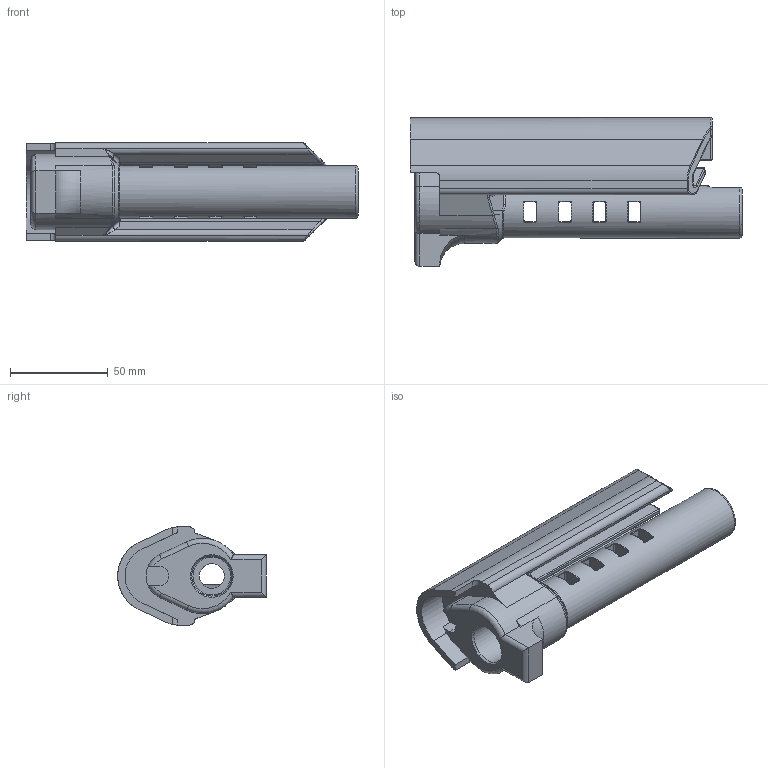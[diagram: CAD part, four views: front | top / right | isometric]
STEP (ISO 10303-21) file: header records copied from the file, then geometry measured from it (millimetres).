
FILE_DESCRIPTION(/* description */ (''),/* implementation_level */ '2;1');
FILE_NAME(/* name */ 'Mount-Cheekrest V2 - Generic.stp',/* time_stamp */ '2021-12-02T15:04:11-06:00',/* author */ ('johne'),/* organization */ (''),/* preprocessor_version */ 'ST-DEVELOPER v18.1',/* originating_system */ 'Autodesk Inventor 2020',/* authorisation */ '');
FILE_SCHEMA (('AUTOMOTIVE_DESIGN { 1 0 10303 214 3 1 1 }'));
Length unit declared in the file: inch
Products named in the file (1): Pho_Spuhr_assembly - Copy
Bounding box: 170.18 x 76.2 x 50.5 mm (x, y, z)
Volume: 191446.3 mm3; surface area: 65570.1 mm2
Topology: 1 solids, 1 shells, 369 faces, 942 edges, 557 vertices
Faces by surface type: cylinder 145, plane 91, bspline 78, torus 49, sphere 4, cone 2
Full cylindrical faces by diameter (mm): 2.75 x1, 12.725 x1, 20.599 x1, 26.924 x1
Entity records: 14156 total; most frequent: CARTESIAN_POINT 5532, ORIENTED_EDGE 1864, DIRECTION 1736, EDGE_CURVE 932, AXIS2_PLACEMENT_3D 687, VERTEX_POINT 557, EDGE_LOOP 381, FACE_OUTER_BOUND 369
